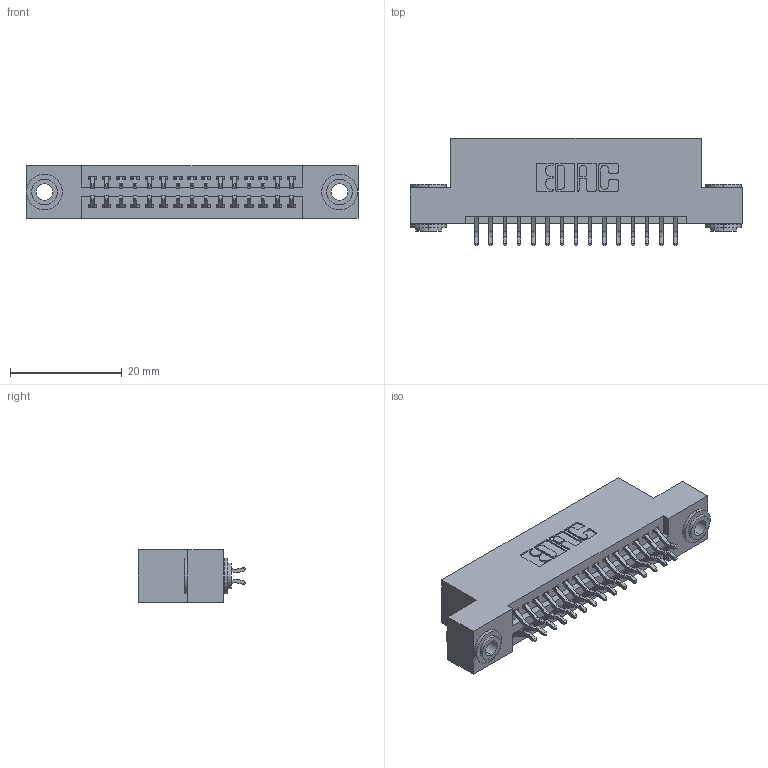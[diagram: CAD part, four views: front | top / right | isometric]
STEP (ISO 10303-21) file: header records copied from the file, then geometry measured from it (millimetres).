
FILE_DESCRIPTION (( 'STEP AP203' ), '1' );
FILE_NAME ('395-030-556-203.STEP', '2018-11-11T07:35:47', ( '' ), ( '' ), 'SwSTEP 2.0', 'SolidWorks 2016', '' );
FILE_SCHEMA (( 'CONFIG_CONTROL_DESIGN' ));
Length unit declared in the file: inch
Products named in the file (4): 345-292-001_556 Tail; 345 Part_Flush Mounting Lugs - 0.156 Dia-TH; 345-250-002_345-250-002-102; 395-030-556-203
Assembly tree (33 placements, depth 2):
  395-030-556-203
    345 Part_Flush Mounting Lugs - 0.156 Dia-TH
    345-292-001_556 Tail  x30
    345-250-002_345-250-002-102  x2
Bounding box: 59.31 x 19.24 x 9.4 mm (x, y, z)
Volume: 5528.9 mm3; surface area: 7828.4 mm2
Topology: 33 solids, 33 shells, 1844 faces, 5427 edges, 3574 vertices
Faces by surface type: plane 1200, cylinder 636, cone 8
Entity records: 16274 total; most frequent: CARTESIAN_POINT 2743, ORIENTED_EDGE 2658, DIRECTION 2471, EDGE_CURVE 1329, VECTOR 1105, LINE 1105, VERTEX_POINT 882, AXIS2_PLACEMENT_3D 683
